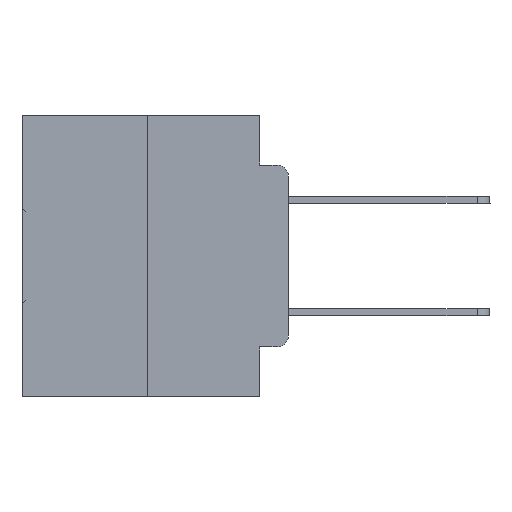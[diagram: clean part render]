
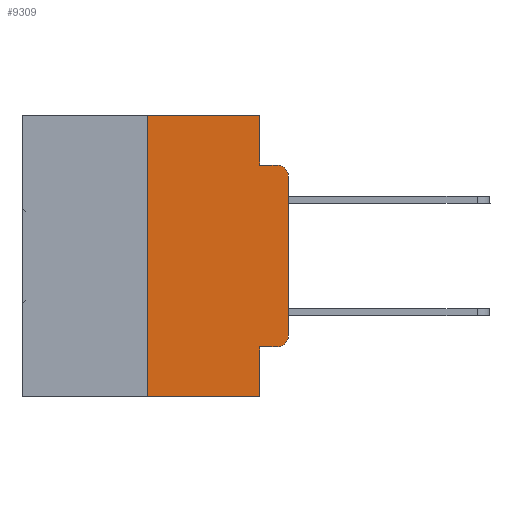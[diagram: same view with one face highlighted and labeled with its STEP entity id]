
A CAD part, left-side view. The second image highlights one B-rep face of the part: STEP entity #9309.
In plain terms, the highlighted planar face has unit normal (-1, 0, 0).
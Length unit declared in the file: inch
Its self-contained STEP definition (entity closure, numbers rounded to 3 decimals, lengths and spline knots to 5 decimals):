
#477 = CARTESIAN_POINT ( 'NONE',  ( 0., 0.051, 0. ) ) ;
#1742 = FACE_OUTER_BOUND ( 'NONE', #14139, .T. ) ;
#2781 = DIRECTION ( 'NONE',  ( 0., 0., 1. ) ) ;
#2865 = ORIENTED_EDGE ( 'NONE', *, *, #3063, .T. ) ;
#3055 = DIRECTION ( 'NONE',  ( -1., 0., 0. ) ) ;
#3063 = EDGE_CURVE ( 'NONE', #8696, #30838, #30162, .T. ) ;
#3586 = CARTESIAN_POINT ( 'NONE',  ( 0., 0.473, 0. ) ) ;
#4090 = ORIENTED_EDGE ( 'NONE', *, *, #9235, .T. ) ;
#4145 = VECTOR ( 'NONE', #14587, 39.37008 ) ;
#4683 = VERTEX_POINT ( 'NONE', #14406 ) ;
#4823 = CARTESIAN_POINT ( 'NONE',  ( 0., 0., -0.3915 ) ) ;
#5170 = VERTEX_POINT ( 'NONE', #30957 ) ;
#5241 = AXIS2_PLACEMENT_3D ( 'NONE', #28386, #3055, #8278 ) ;
#5384 = CARTESIAN_POINT ( 'NONE',  ( 0., 0.02, -0.0885 ) ) ;
#5400 = ORIENTED_EDGE ( 'NONE', *, *, #31606, .T. ) ;
#6001 = AXIS2_PLACEMENT_3D ( 'NONE', #15932, #20646, #20856 ) ;
#6460 = DIRECTION ( 'NONE',  ( 0., 0., -1. ) ) ;
#6518 = VECTOR ( 'NONE', #7103, 39.37008 ) ;
#7103 = DIRECTION ( 'NONE',  ( 0., 0., -1. ) ) ;
#7491 = ORIENTED_EDGE ( 'NONE', *, *, #29869, .T. ) ;
#7729 = VECTOR ( 'NONE', #2781, 39.37008 ) ;
#8252 = CARTESIAN_POINT ( 'NONE',  ( 0., 0.25, 0. ) ) ;
#8278 = DIRECTION ( 'NONE',  ( 0., 0., -1. ) ) ;
#8696 = VERTEX_POINT ( 'NONE', #21805 ) ;
#8708 = ORIENTED_EDGE ( 'NONE', *, *, #16790, .F. ) ;
#9235 = EDGE_CURVE ( 'NONE', #14672, #8696, #21883, .T. ) ;
#9309 = ADVANCED_FACE ( 'NONE', ( #1742 ), #16487, .F. ) ;
#9331 = LINE ( 'NONE', #22770, #7729 ) ;
#10758 = VECTOR ( 'NONE', #32280, 39.37008 ) ;
#11113 = DIRECTION ( 'NONE',  ( 0., -1., 0. ) ) ;
#11639 = CARTESIAN_POINT ( 'NONE',  ( 0., 0.473, 0. ) ) ;
#12051 = CARTESIAN_POINT ( 'NONE',  ( 0., 0.051, 0. ) ) ;
#12174 = DIRECTION ( 'NONE',  ( 0., -1., 0. ) ) ;
#12684 = LINE ( 'NONE', #31109, #25313 ) ;
#12850 = LINE ( 'NONE', #12051, #4145 ) ;
#13574 = VERTEX_POINT ( 'NONE', #27769 ) ;
#13650 = CARTESIAN_POINT ( 'NONE',  ( 0., 0., 0. ) ) ;
#13860 = VERTEX_POINT ( 'NONE', #24089 ) ;
#14049 = EDGE_CURVE ( 'NONE', #19140, #13860, #12850, .T. ) ;
#14139 = EDGE_LOOP ( 'NONE', ( #4090, #2865, #19358, #21355, #8708, #17064, #14475, #20229, #7491, #5400 ) ) ;
#14406 = CARTESIAN_POINT ( 'NONE',  ( 0., 0.25, -0.5 ) ) ;
#14475 = ORIENTED_EDGE ( 'NONE', *, *, #30040, .T. ) ;
#14587 = DIRECTION ( 'NONE',  ( 0., 0., -1. ) ) ;
#14672 = VERTEX_POINT ( 'NONE', #4823 ) ;
#15612 = LINE ( 'NONE', #26566, #6518 ) ;
#15932 = CARTESIAN_POINT ( 'NONE',  ( 0., 0.02, -0.3915 ) ) ;
#16487 = PLANE ( 'NONE',  #30987 ) ;
#16790 = EDGE_CURVE ( 'NONE', #21561, #19140, #30445, .T. ) ;
#17064 = ORIENTED_EDGE ( 'NONE', *, *, #19149, .F. ) ;
#18242 = VECTOR ( 'NONE', #12174, 39.37008 ) ;
#18630 = LINE ( 'NONE', #29749, #10758 ) ;
#18882 = CARTESIAN_POINT ( 'NONE',  ( 0., 0.051, -0.4115 ) ) ;
#19140 = VERTEX_POINT ( 'NONE', #477 ) ;
#19149 = EDGE_CURVE ( 'NONE', #4683, #21561, #9331, .T. ) ;
#19241 = DIRECTION ( 'NONE',  ( 1., 0., 0. ) ) ;
#19358 = ORIENTED_EDGE ( 'NONE', *, *, #30977, .F. ) ;
#20229 = ORIENTED_EDGE ( 'NONE', *, *, #27937, .F. ) ;
#20646 = DIRECTION ( 'NONE',  ( -1., 0., 0. ) ) ;
#20856 = DIRECTION ( 'NONE',  ( 0., 0., -1. ) ) ;
#21355 = ORIENTED_EDGE ( 'NONE', *, *, #14049, .F. ) ;
#21561 = VERTEX_POINT ( 'NONE', #8252 ) ;
#21805 = CARTESIAN_POINT ( 'NONE',  ( 0., 0., -0.1085 ) ) ;
#21883 = LINE ( 'NONE', #13650, #27869 ) ;
#22491 = VECTOR ( 'NONE', #11113, 39.37008 ) ;
#22770 = CARTESIAN_POINT ( 'NONE',  ( 0., 0.25, 0. ) ) ;
#24089 = CARTESIAN_POINT ( 'NONE',  ( 0., 0.051, -0.0885 ) ) ;
#24994 = LINE ( 'NONE', #18882, #18242 ) ;
#25313 = VECTOR ( 'NONE', #25593, 39.37008 ) ;
#25593 = DIRECTION ( 'NONE',  ( 0., -1., 0. ) ) ;
#26232 = DIRECTION ( 'NONE',  ( 0., 0., 1. ) ) ;
#26566 = CARTESIAN_POINT ( 'NONE',  ( 0., 0.051, 0. ) ) ;
#27769 = CARTESIAN_POINT ( 'NONE',  ( 0., 0.051, -0.4115 ) ) ;
#27869 = VECTOR ( 'NONE', #26232, 39.37008 ) ;
#27937 = EDGE_CURVE ( 'NONE', #13574, #5170, #15612, .T. ) ;
#28055 = CIRCLE ( 'NONE', #6001, 0.02 ) ;
#28386 = CARTESIAN_POINT ( 'NONE',  ( 0., 0.02, -0.1085 ) ) ;
#29265 = VERTEX_POINT ( 'NONE', #31750 ) ;
#29749 = CARTESIAN_POINT ( 'NONE',  ( 0., 0.473, -0.5 ) ) ;
#29869 = EDGE_CURVE ( 'NONE', #13574, #29265, #24994, .T. ) ;
#30040 = EDGE_CURVE ( 'NONE', #4683, #5170, #18630, .T. ) ;
#30162 = CIRCLE ( 'NONE', #5241, 0.02 ) ;
#30445 = LINE ( 'NONE', #3586, #22491 ) ;
#30838 = VERTEX_POINT ( 'NONE', #5384 ) ;
#30957 = CARTESIAN_POINT ( 'NONE',  ( 0., 0.051, -0.5 ) ) ;
#30977 = EDGE_CURVE ( 'NONE', #13860, #30838, #12684, .T. ) ;
#30987 = AXIS2_PLACEMENT_3D ( 'NONE', #11639, #19241, #6460 ) ;
#31109 = CARTESIAN_POINT ( 'NONE',  ( 0., 0.051, -0.0885 ) ) ;
#31606 = EDGE_CURVE ( 'NONE', #29265, #14672, #28055, .T. ) ;
#31750 = CARTESIAN_POINT ( 'NONE',  ( 0., 0.02, -0.4115 ) ) ;
#32280 = DIRECTION ( 'NONE',  ( 0., -1., 0. ) ) ;
